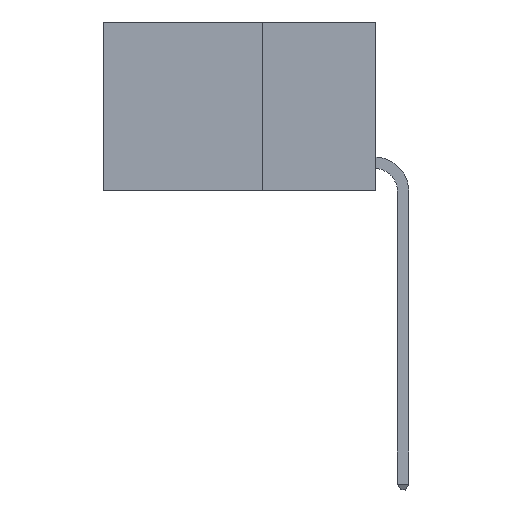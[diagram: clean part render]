
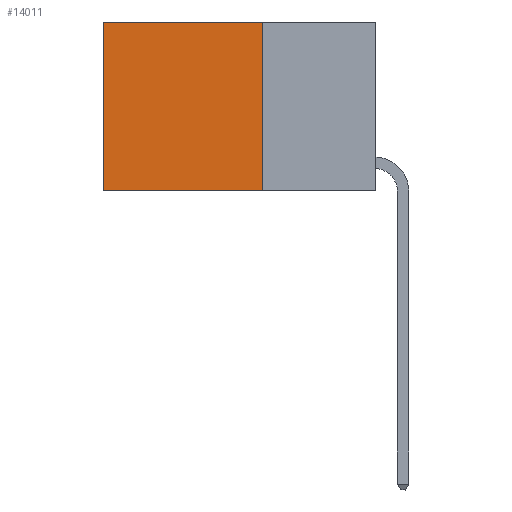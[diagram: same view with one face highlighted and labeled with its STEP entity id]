
A CAD part, left-side view. The second image highlights one B-rep face of the part: STEP entity #14011.
In plain terms, the highlighted planar face has unit normal (-1, 0, 0).
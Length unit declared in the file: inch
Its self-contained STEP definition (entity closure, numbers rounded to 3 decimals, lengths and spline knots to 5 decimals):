
#1044 = CARTESIAN_POINT ( 'NONE',  ( 0.2625, 0.25, 0. ) ) ;
#1883 = LINE ( 'NONE', #18821, #19141 ) ;
#2018 = CARTESIAN_POINT ( 'NONE',  ( 0.2625, 0.25, 0. ) ) ;
#4296 = DIRECTION ( 'NONE',  ( 0., 0., -1. ) ) ;
#5118 = CARTESIAN_POINT ( 'NONE',  ( 0.2625, 0.6, -0.37 ) ) ;
#5284 = CARTESIAN_POINT ( 'NONE',  ( 0.2625, 0.6, 0. ) ) ;
#5404 = EDGE_CURVE ( 'NONE', #19514, #23649, #14029, .T. ) ;
#6701 = CARTESIAN_POINT ( 'NONE',  ( 0.2625, 0.6, 0. ) ) ;
#10127 = EDGE_CURVE ( 'NONE', #26309, #24972, #1883, .T. ) ;
#10963 = CARTESIAN_POINT ( 'NONE',  ( 0.2625, 0.25, 0. ) ) ;
#12207 = ORIENTED_EDGE ( 'NONE', *, *, #10127, .F. ) ;
#12569 = LINE ( 'NONE', #10963, #23717 ) ;
#12713 = LINE ( 'NONE', #6701, #17898 ) ;
#12739 = CARTESIAN_POINT ( 'NONE',  ( 0.2625, 0.25, 0. ) ) ;
#13229 = DIRECTION ( 'NONE',  ( 0., 0., -1. ) ) ;
#13335 = VECTOR ( 'NONE', #28022, 39.37008 ) ;
#14011 = ADVANCED_FACE ( 'NONE', ( #20701 ), #26620, .F. ) ;
#14029 = LINE ( 'NONE', #1044, #13335 ) ;
#14878 = ORIENTED_EDGE ( 'NONE', *, *, #25314, .F. ) ;
#16717 = ORIENTED_EDGE ( 'NONE', *, *, #5404, .T. ) ;
#17215 = EDGE_CURVE ( 'NONE', #23649, #24972, #12713, .T. ) ;
#17762 = DIRECTION ( 'NONE',  ( 1., 0., 0. ) ) ;
#17898 = VECTOR ( 'NONE', #22477, 39.37008 ) ;
#18821 = CARTESIAN_POINT ( 'NONE',  ( 0.2625, 0.25, -0.37 ) ) ;
#19141 = VECTOR ( 'NONE', #27783, 39.37008 ) ;
#19514 = VERTEX_POINT ( 'NONE', #12739 ) ;
#19534 = CARTESIAN_POINT ( 'NONE',  ( 0.2625, 0.25, -0.37 ) ) ;
#19770 = AXIS2_PLACEMENT_3D ( 'NONE', #2018, #17762, #4296 ) ;
#20340 = EDGE_LOOP ( 'NONE', ( #28720, #12207, #14878, #16717 ) ) ;
#20701 = FACE_OUTER_BOUND ( 'NONE', #20340, .T. ) ;
#22477 = DIRECTION ( 'NONE',  ( 0., 0., -1. ) ) ;
#23649 = VERTEX_POINT ( 'NONE', #5284 ) ;
#23717 = VECTOR ( 'NONE', #13229, 39.37008 ) ;
#24972 = VERTEX_POINT ( 'NONE', #5118 ) ;
#25314 = EDGE_CURVE ( 'NONE', #19514, #26309, #12569, .T. ) ;
#26309 = VERTEX_POINT ( 'NONE', #19534 ) ;
#26620 = PLANE ( 'NONE',  #19770 ) ;
#27783 = DIRECTION ( 'NONE',  ( 0., 1., 0. ) ) ;
#28022 = DIRECTION ( 'NONE',  ( 0., 1., 0. ) ) ;
#28720 = ORIENTED_EDGE ( 'NONE', *, *, #17215, .T. ) ;
